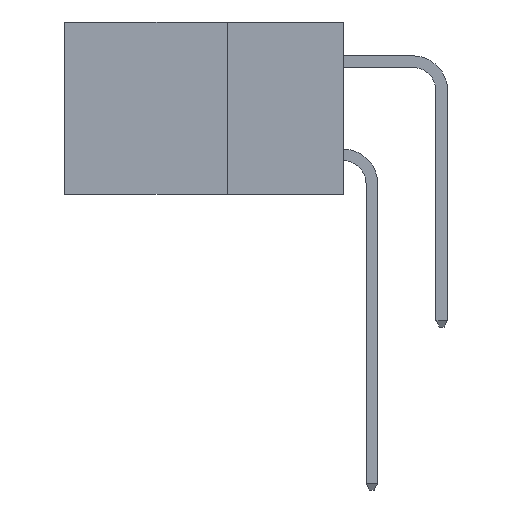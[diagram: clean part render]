
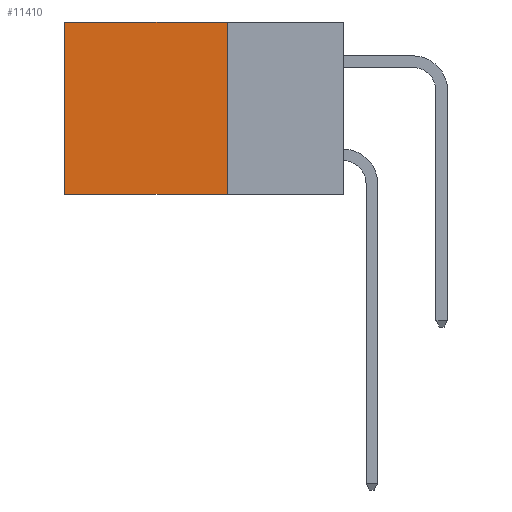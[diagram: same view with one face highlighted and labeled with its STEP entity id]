
A CAD part, left-side view. The second image highlights one B-rep face of the part: STEP entity #11410.
In plain terms, the highlighted planar face has unit normal (-1, 0, 0).
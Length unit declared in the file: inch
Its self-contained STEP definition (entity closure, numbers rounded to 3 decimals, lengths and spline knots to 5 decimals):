
#183 = DIRECTION ( 'NONE',  ( 0., 0., -1. ) ) ;
#1150 = ORIENTED_EDGE ( 'NONE', *, *, #7257, .T. ) ;
#1481 = DIRECTION ( 'NONE',  ( 0., 0., -1. ) ) ;
#1693 = ORIENTED_EDGE ( 'NONE', *, *, #11879, .T. ) ;
#2172 = DIRECTION ( 'NONE',  ( 1., 0., 0. ) ) ;
#2612 = CARTESIAN_POINT ( 'NONE',  ( 0.2615, 0.6, 0. ) ) ;
#2679 = EDGE_CURVE ( 'NONE', #5453, #11531, #12111, .T. ) ;
#3319 = VECTOR ( 'NONE', #183, 39.37008 ) ;
#4160 = VECTOR ( 'NONE', #17883, 39.37008 ) ;
#4530 = VERTEX_POINT ( 'NONE', #2612 ) ;
#5306 = EDGE_LOOP ( 'NONE', ( #1693, #13849, #6513, #1150 ) ) ;
#5370 = CARTESIAN_POINT ( 'NONE',  ( 0.2615, 0.6, -0.37 ) ) ;
#5453 = VERTEX_POINT ( 'NONE', #10700 ) ;
#6513 = ORIENTED_EDGE ( 'NONE', *, *, #11043, .F. ) ;
#7236 = CARTESIAN_POINT ( 'NONE',  ( 0.2615, 0.25, 0. ) ) ;
#7257 = EDGE_CURVE ( 'NONE', #13519, #4530, #16546, .T. ) ;
#9424 = VECTOR ( 'NONE', #1481, 39.37008 ) ;
#10344 = CARTESIAN_POINT ( 'NONE',  ( 0.2615, 0.25, -0.37 ) ) ;
#10640 = CARTESIAN_POINT ( 'NONE',  ( 0.2615, 0.6, -0.37 ) ) ;
#10700 = CARTESIAN_POINT ( 'NONE',  ( 0.2615, 0.25, -0.37 ) ) ;
#11043 = EDGE_CURVE ( 'NONE', #13519, #5453, #13403, .T. ) ;
#11124 = CARTESIAN_POINT ( 'NONE',  ( 0.2615, 0.25, -0.37 ) ) ;
#11386 = CARTESIAN_POINT ( 'NONE',  ( 0.2615, 0.25, 0. ) ) ;
#11410 = ADVANCED_FACE ( 'NONE', ( #16131 ), #18460, .F. ) ;
#11531 = VERTEX_POINT ( 'NONE', #5370 ) ;
#11627 = DIRECTION ( 'NONE',  ( 0., 1., 0. ) ) ;
#11879 = EDGE_CURVE ( 'NONE', #4530, #11531, #18185, .T. ) ;
#12111 = LINE ( 'NONE', #17863, #4160 ) ;
#12628 = DIRECTION ( 'NONE',  ( 0., 0., -1. ) ) ;
#13403 = LINE ( 'NONE', #10344, #9424 ) ;
#13519 = VERTEX_POINT ( 'NONE', #11386 ) ;
#13849 = ORIENTED_EDGE ( 'NONE', *, *, #2679, .F. ) ;
#16131 = FACE_OUTER_BOUND ( 'NONE', #5306, .T. ) ;
#16137 = AXIS2_PLACEMENT_3D ( 'NONE', #11124, #2172, #12628 ) ;
#16546 = LINE ( 'NONE', #7236, #19085 ) ;
#17863 = CARTESIAN_POINT ( 'NONE',  ( 0.2615, 0.25, -0.37 ) ) ;
#17883 = DIRECTION ( 'NONE',  ( 0., 1., 0. ) ) ;
#18185 = LINE ( 'NONE', #10640, #3319 ) ;
#18460 = PLANE ( 'NONE',  #16137 ) ;
#19085 = VECTOR ( 'NONE', #11627, 39.37008 ) ;
